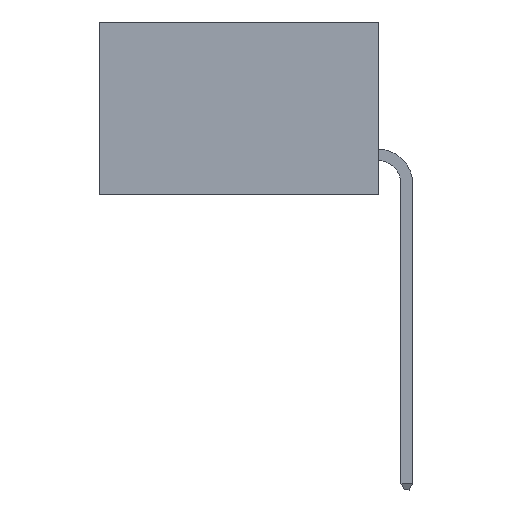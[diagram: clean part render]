
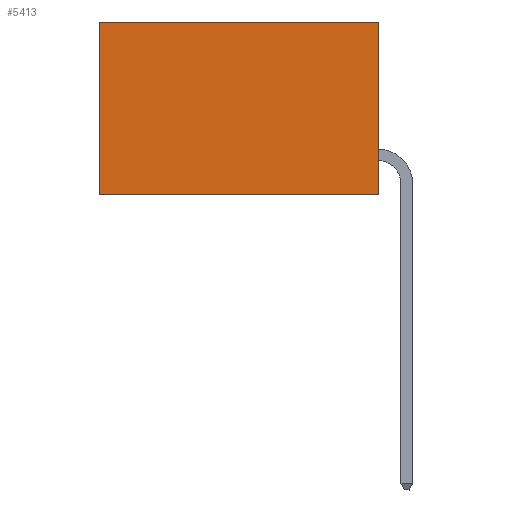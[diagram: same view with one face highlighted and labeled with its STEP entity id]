
A CAD part, left-side view. The second image highlights one B-rep face of the part: STEP entity #5413.
In plain terms, the highlighted planar face has unit normal (-1, 0, 0).
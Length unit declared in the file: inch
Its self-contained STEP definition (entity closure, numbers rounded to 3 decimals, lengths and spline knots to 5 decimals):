
#737 = CARTESIAN_POINT ( 'NONE',  ( 0.298, 0.6, 0. ) ) ;
#1040 = DIRECTION ( 'NONE',  ( 0., 1., 0. ) ) ;
#1303 = CARTESIAN_POINT ( 'NONE',  ( 0.298, 0., 0. ) ) ;
#2067 = ORIENTED_EDGE ( 'NONE', *, *, #8083, .F. ) ;
#2527 = DIRECTION ( 'NONE',  ( 1., 0., 0. ) ) ;
#3365 = LINE ( 'NONE', #737, #13676 ) ;
#4240 = DIRECTION ( 'NONE',  ( 0., 0., -1. ) ) ;
#4339 = AXIS2_PLACEMENT_3D ( 'NONE', #9865, #2527, #14601 ) ;
#4647 = LINE ( 'NONE', #17134, #9070 ) ;
#5152 = LINE ( 'NONE', #9184, #9147 ) ;
#5286 = EDGE_CURVE ( 'NONE', #11732, #10659, #3365, .T. ) ;
#5413 = ADVANCED_FACE ( 'NONE', ( #15148 ), #9363, .F. ) ;
#5672 = CARTESIAN_POINT ( 'NONE',  ( 0.298, 0., 0. ) ) ;
#6523 = ORIENTED_EDGE ( 'NONE', *, *, #5286, .T. ) ;
#7100 = CARTESIAN_POINT ( 'NONE',  ( 0.298, 0.6, -0.37 ) ) ;
#7303 = DIRECTION ( 'NONE',  ( 0., 0., -1. ) ) ;
#8083 = EDGE_CURVE ( 'NONE', #15212, #16486, #16130, .T. ) ;
#8962 = VECTOR ( 'NONE', #4240, 39.37008 ) ;
#9070 = VECTOR ( 'NONE', #9092, 39.37008 ) ;
#9092 = DIRECTION ( 'NONE',  ( 0., 1., 0. ) ) ;
#9147 = VECTOR ( 'NONE', #1040, 39.37008 ) ;
#9184 = CARTESIAN_POINT ( 'NONE',  ( 0.298, 0., 0. ) ) ;
#9363 = PLANE ( 'NONE',  #4339 ) ;
#9711 = EDGE_CURVE ( 'NONE', #15212, #11732, #5152, .T. ) ;
#9865 = CARTESIAN_POINT ( 'NONE',  ( 0.298, 0., 0. ) ) ;
#10659 = VERTEX_POINT ( 'NONE', #7100 ) ;
#11732 = VERTEX_POINT ( 'NONE', #11936 ) ;
#11936 = CARTESIAN_POINT ( 'NONE',  ( 0.298, 0.6, 0. ) ) ;
#12544 = EDGE_LOOP ( 'NONE', ( #6523, #14238, #2067, #13687 ) ) ;
#13487 = CARTESIAN_POINT ( 'NONE',  ( 0.298, 0., -0.37 ) ) ;
#13676 = VECTOR ( 'NONE', #7303, 39.37008 ) ;
#13687 = ORIENTED_EDGE ( 'NONE', *, *, #9711, .T. ) ;
#14238 = ORIENTED_EDGE ( 'NONE', *, *, #16399, .F. ) ;
#14601 = DIRECTION ( 'NONE',  ( 0., 0., -1. ) ) ;
#15148 = FACE_OUTER_BOUND ( 'NONE', #12544, .T. ) ;
#15212 = VERTEX_POINT ( 'NONE', #1303 ) ;
#16130 = LINE ( 'NONE', #5672, #8962 ) ;
#16399 = EDGE_CURVE ( 'NONE', #16486, #10659, #4647, .T. ) ;
#16486 = VERTEX_POINT ( 'NONE', #13487 ) ;
#17134 = CARTESIAN_POINT ( 'NONE',  ( 0.298, 0., -0.37 ) ) ;
